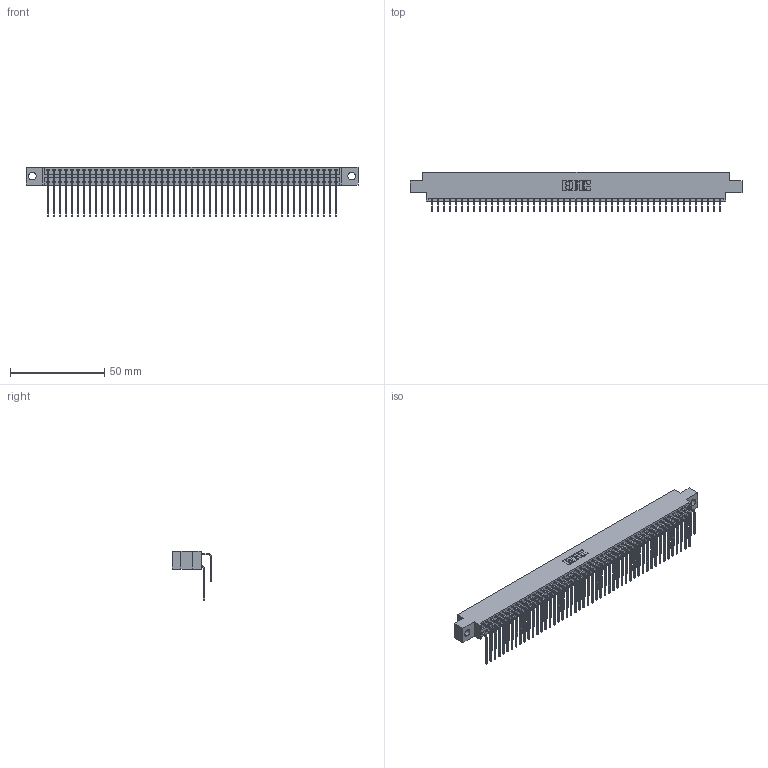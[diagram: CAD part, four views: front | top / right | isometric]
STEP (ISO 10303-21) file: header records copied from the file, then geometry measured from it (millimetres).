
FILE_DESCRIPTION (( 'STEP AP203' ), '1' );
FILE_NAME ('396-098-559-804.STEP', '2018-09-14T06:06:23', ( '' ), ( '' ), 'SwSTEP 2.0', 'SolidWorks 2016', '' );
FILE_SCHEMA (( 'CONFIG_CONTROL_DESIGN' ));
Length unit declared in the file: inch
Products named in the file (4): 396-098-559-804; 346 Part_0.170 Offset - 0.156 Dia-TH; 345-292-001_558 559 Tail - 1; 345-292-001_559 Tail - 2
Assembly tree (99 placements, depth 2):
  396-098-559-804
    346 Part_0.170 Offset - 0.156 Dia-TH
    345-292-001_558 559 Tail - 1  x49
    345-292-001_559 Tail - 2  x49
Bounding box: 176.15 x 20.89 x 26.16 mm (x, y, z)
Volume: 17553.9 mm3; surface area: 26944.2 mm2
Topology: 99 solids, 99 shells, 5418 faces, 16119 edges, 10614 vertices
Faces by surface type: plane 3706, cylinder 1712
Entity records: 32955 total; most frequent: CARTESIAN_POINT 5475, ORIENTED_EDGE 5358, DIRECTION 4847, EDGE_CURVE 2679, LINE 2311, VECTOR 2311, VERTEX_POINT 1782, AXIS2_PLACEMENT_3D 1268
